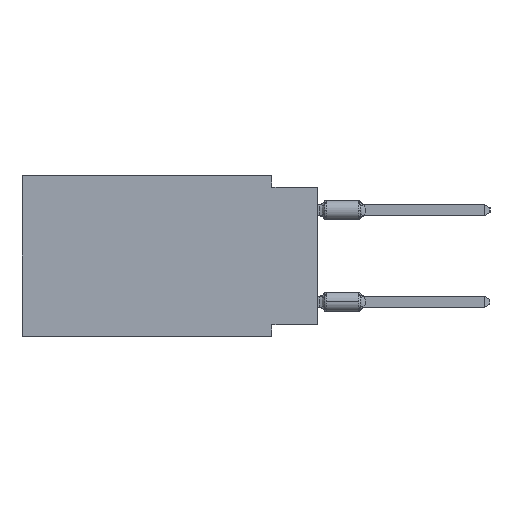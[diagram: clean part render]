
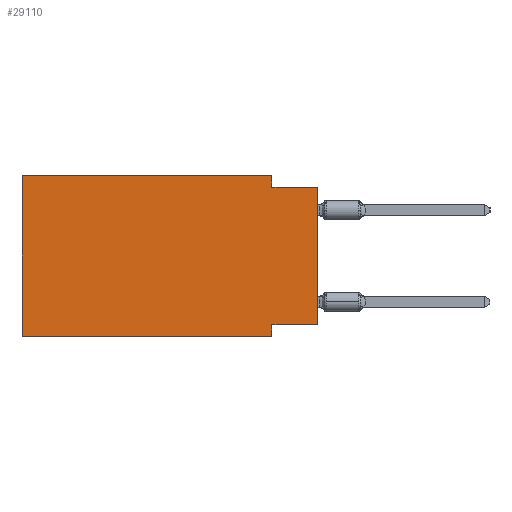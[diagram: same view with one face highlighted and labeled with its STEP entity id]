
A CAD part, left-side view. The second image highlights one B-rep face of the part: STEP entity #29110.
In plain terms, the highlighted planar face has unit normal (-1, 0, 0).
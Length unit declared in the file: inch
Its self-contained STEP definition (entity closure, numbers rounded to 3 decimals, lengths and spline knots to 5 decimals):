
#640 = LINE ( 'NONE', #22084, #8499 ) ;
#757 = DIRECTION ( 'NONE',  ( 0., 0., -1. ) ) ;
#1100 = DIRECTION ( 'NONE',  ( 0., -1., 0. ) ) ;
#1426 = DIRECTION ( 'NONE',  ( 0., 0., -1. ) ) ;
#1476 = LINE ( 'NONE', #10712, #30510 ) ;
#1874 = LINE ( 'NONE', #4809, #34615 ) ;
#1880 = DIRECTION ( 'NONE',  ( 0., 0., 1. ) ) ;
#1990 = CARTESIAN_POINT ( 'NONE',  ( 0., 0., -0.325 ) ) ;
#2789 = VERTEX_POINT ( 'NONE', #5321 ) ;
#4272 = VERTEX_POINT ( 'NONE', #6314 ) ;
#4809 = CARTESIAN_POINT ( 'NONE',  ( 0., 0.645, 0. ) ) ;
#4866 = LINE ( 'NONE', #37131, #15421 ) ;
#5321 = CARTESIAN_POINT ( 'NONE',  ( 0., 0., -0.025 ) ) ;
#6314 = CARTESIAN_POINT ( 'NONE',  ( 0., 0.1, -0.35 ) ) ;
#8499 = VECTOR ( 'NONE', #12642, 39.37008 ) ;
#8515 = EDGE_CURVE ( 'NONE', #34853, #16560, #19073, .T. ) ;
#9693 = ORIENTED_EDGE ( 'NONE', *, *, #20168, .F. ) ;
#9836 = ORIENTED_EDGE ( 'NONE', *, *, #11711, .F. ) ;
#10606 = VECTOR ( 'NONE', #21277, 39.37008 ) ;
#10712 = CARTESIAN_POINT ( 'NONE',  ( 0., 0., 0. ) ) ;
#11711 = EDGE_CURVE ( 'NONE', #23318, #2789, #4866, .T. ) ;
#12071 = EDGE_CURVE ( 'NONE', #13792, #2789, #1476, .T. ) ;
#12173 = CARTESIAN_POINT ( 'NONE',  ( 0., 0.645, 0. ) ) ;
#12642 = DIRECTION ( 'NONE',  ( 0., -1., 0. ) ) ;
#12925 = CARTESIAN_POINT ( 'NONE',  ( 0., 0.1, -0.325 ) ) ;
#13792 = VERTEX_POINT ( 'NONE', #21743 ) ;
#14002 = DIRECTION ( 'NONE',  ( 0., 1., 0. ) ) ;
#15367 = ORIENTED_EDGE ( 'NONE', *, *, #23604, .F. ) ;
#15421 = VECTOR ( 'NONE', #31449, 39.37008 ) ;
#16009 = CARTESIAN_POINT ( 'NONE',  ( 0., 0.645, -0.35 ) ) ;
#16024 = ORIENTED_EDGE ( 'NONE', *, *, #8515, .F. ) ;
#16509 = ORIENTED_EDGE ( 'NONE', *, *, #30049, .F. ) ;
#16560 = VERTEX_POINT ( 'NONE', #17229 ) ;
#17121 = AXIS2_PLACEMENT_3D ( 'NONE', #12173, #36748, #757 ) ;
#17229 = CARTESIAN_POINT ( 'NONE',  ( 0., 0.645, 0. ) ) ;
#19073 = LINE ( 'NONE', #30708, #23659 ) ;
#20168 = EDGE_CURVE ( 'NONE', #13792, #33293, #28957, .T. ) ;
#20939 = VERTEX_POINT ( 'NONE', #26876 ) ;
#21052 = FACE_OUTER_BOUND ( 'NONE', #31091, .T. ) ;
#21277 = DIRECTION ( 'NONE',  ( 0., 0., -1. ) ) ;
#21516 = EDGE_CURVE ( 'NONE', #34853, #4272, #640, .T. ) ;
#21743 = CARTESIAN_POINT ( 'NONE',  ( 0., 0., -0.325 ) ) ;
#22084 = CARTESIAN_POINT ( 'NONE',  ( 0., 0.645, -0.35 ) ) ;
#23318 = VERTEX_POINT ( 'NONE', #35771 ) ;
#23604 = EDGE_CURVE ( 'NONE', #20939, #23318, #38783, .T. ) ;
#23659 = VECTOR ( 'NONE', #28512, 39.37008 ) ;
#23975 = PLANE ( 'NONE',  #17121 ) ;
#24871 = ORIENTED_EDGE ( 'NONE', *, *, #12071, .T. ) ;
#25304 = VECTOR ( 'NONE', #1426, 39.37008 ) ;
#26779 = CARTESIAN_POINT ( 'NONE',  ( 0., 0.1, 0. ) ) ;
#26876 = CARTESIAN_POINT ( 'NONE',  ( 0., 0.1, 0. ) ) ;
#27386 = EDGE_CURVE ( 'NONE', #16560, #20939, #1874, .T. ) ;
#27422 = ORIENTED_EDGE ( 'NONE', *, *, #21516, .T. ) ;
#28391 = CARTESIAN_POINT ( 'NONE',  ( 0., 0.1, -0.35 ) ) ;
#28512 = DIRECTION ( 'NONE',  ( 0., 0., 1. ) ) ;
#28957 = LINE ( 'NONE', #1990, #34830 ) ;
#29110 = ADVANCED_FACE ( 'NONE', ( #21052 ), #23975, .F. ) ;
#30049 = EDGE_CURVE ( 'NONE', #33293, #4272, #34083, .T. ) ;
#30510 = VECTOR ( 'NONE', #1880, 39.37008 ) ;
#30708 = CARTESIAN_POINT ( 'NONE',  ( 0., 0.645, 0. ) ) ;
#31091 = EDGE_LOOP ( 'NONE', ( #24871, #9836, #15367, #35154, #16024, #27422, #16509, #9693 ) ) ;
#31449 = DIRECTION ( 'NONE',  ( 0., -1., 0. ) ) ;
#33293 = VERTEX_POINT ( 'NONE', #12925 ) ;
#34083 = LINE ( 'NONE', #28391, #25304 ) ;
#34615 = VECTOR ( 'NONE', #1100, 39.37008 ) ;
#34830 = VECTOR ( 'NONE', #14002, 39.37008 ) ;
#34853 = VERTEX_POINT ( 'NONE', #16009 ) ;
#35154 = ORIENTED_EDGE ( 'NONE', *, *, #27386, .F. ) ;
#35771 = CARTESIAN_POINT ( 'NONE',  ( 0., 0.1, -0.025 ) ) ;
#36748 = DIRECTION ( 'NONE',  ( 1., 0., 0. ) ) ;
#37131 = CARTESIAN_POINT ( 'NONE',  ( 0., 0., -0.025 ) ) ;
#38783 = LINE ( 'NONE', #26779, #10606 ) ;
